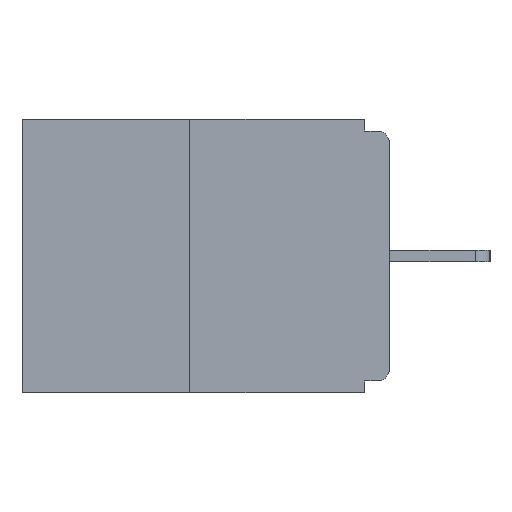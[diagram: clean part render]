
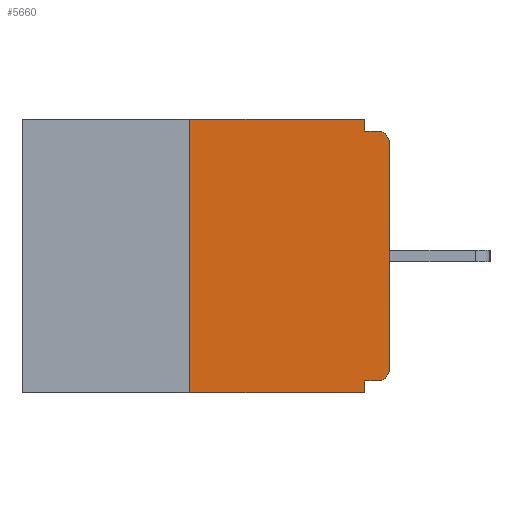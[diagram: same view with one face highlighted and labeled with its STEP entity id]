
A CAD part, left-side view. The second image highlights one B-rep face of the part: STEP entity #5660.
In plain terms, the highlighted planar face has unit normal (-1, 0, 0).
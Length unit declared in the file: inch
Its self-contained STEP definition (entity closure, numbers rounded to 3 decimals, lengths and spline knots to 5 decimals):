
#45 = ORIENTED_EDGE ( 'NONE', *, *, #11676, .F. ) ;
#504 = VECTOR ( 'NONE', #8665, 39.37008 ) ;
#790 = DIRECTION ( 'NONE',  ( 0., -1., 0. ) ) ;
#832 = CARTESIAN_POINT ( 'NONE',  ( 0., 0.46, 0. ) ) ;
#844 = CARTESIAN_POINT ( 'NONE',  ( 0., 0.031, -0.343 ) ) ;
#902 = PLANE ( 'NONE',  #1967 ) ;
#1046 = VERTEX_POINT ( 'NONE', #8245 ) ;
#1131 = LINE ( 'NONE', #14130, #15186 ) ;
#1216 = ORIENTED_EDGE ( 'NONE', *, *, #13481, .F. ) ;
#1357 = CARTESIAN_POINT ( 'NONE',  ( 0., 0.031, -0.015 ) ) ;
#1545 = ORIENTED_EDGE ( 'NONE', *, *, #9710, .T. ) ;
#1563 = LINE ( 'NONE', #6252, #3145 ) ;
#1680 = EDGE_CURVE ( 'NONE', #12583, #5940, #13555, .T. ) ;
#1902 = CARTESIAN_POINT ( 'NONE',  ( 0., 0.25, -0.343 ) ) ;
#1910 = CARTESIAN_POINT ( 'NONE',  ( 0., 0.015, -0.015 ) ) ;
#1967 = AXIS2_PLACEMENT_3D ( 'NONE', #832, #1994, #3025 ) ;
#1988 = CARTESIAN_POINT ( 'NONE',  ( 0., 0., 0. ) ) ;
#1994 = DIRECTION ( 'NONE',  ( 1., 0., 0. ) ) ;
#2125 = DIRECTION ( 'NONE',  ( 0., 0., -1. ) ) ;
#2449 = VECTOR ( 'NONE', #7074, 39.37008 ) ;
#2822 = CARTESIAN_POINT ( 'NONE',  ( 0., 0.031, 0. ) ) ;
#3025 = DIRECTION ( 'NONE',  ( 0., 0., -1. ) ) ;
#3145 = VECTOR ( 'NONE', #12181, 39.37008 ) ;
#3301 = DIRECTION ( 'NONE',  ( -1., 0., 0. ) ) ;
#3336 = DIRECTION ( 'NONE',  ( 0., 0., -1. ) ) ;
#3425 = CARTESIAN_POINT ( 'NONE',  ( 0., 0., -0.03 ) ) ;
#3451 = DIRECTION ( 'NONE',  ( -1., 0., 0. ) ) ;
#3454 = EDGE_CURVE ( 'NONE', #7929, #8528, #11336, .T. ) ;
#3764 = VECTOR ( 'NONE', #10218, 39.37008 ) ;
#3963 = VERTEX_POINT ( 'NONE', #1902 ) ;
#4091 = CARTESIAN_POINT ( 'NONE',  ( 0., 0.031, 0. ) ) ;
#4121 = CARTESIAN_POINT ( 'NONE',  ( 0., 0.46, 0. ) ) ;
#4866 = CARTESIAN_POINT ( 'NONE',  ( 0., 0.015, -0.328 ) ) ;
#4900 = CIRCLE ( 'NONE', #6665, 0.015 ) ;
#5142 = VERTEX_POINT ( 'NONE', #1910 ) ;
#5660 = ADVANCED_FACE ( 'NONE', ( #11461 ), #902, .F. ) ;
#5722 = CARTESIAN_POINT ( 'NONE',  ( 0., 0.015, -0.313 ) ) ;
#5940 = VERTEX_POINT ( 'NONE', #1357 ) ;
#6252 = CARTESIAN_POINT ( 'NONE',  ( 0., 0.25, 0. ) ) ;
#6557 = CARTESIAN_POINT ( 'NONE',  ( 0., 0.031, -0.328 ) ) ;
#6665 = AXIS2_PLACEMENT_3D ( 'NONE', #9496, #3451, #2125 ) ;
#7074 = DIRECTION ( 'NONE',  ( 0., 0., 1. ) ) ;
#7313 = VECTOR ( 'NONE', #3336, 39.37008 ) ;
#7446 = VECTOR ( 'NONE', #790, 39.37008 ) ;
#7634 = ORIENTED_EDGE ( 'NONE', *, *, #10480, .T. ) ;
#7929 = VERTEX_POINT ( 'NONE', #6557 ) ;
#8245 = CARTESIAN_POINT ( 'NONE',  ( 0., 0.25, 0. ) ) ;
#8295 = ORIENTED_EDGE ( 'NONE', *, *, #1680, .F. ) ;
#8528 = VERTEX_POINT ( 'NONE', #12852 ) ;
#8605 = EDGE_CURVE ( 'NONE', #11984, #7929, #9116, .T. ) ;
#8665 = DIRECTION ( 'NONE',  ( 0., -1., 0. ) ) ;
#8825 = LINE ( 'NONE', #4121, #504 ) ;
#9088 = DIRECTION ( 'NONE',  ( 0., 0., -1. ) ) ;
#9116 = LINE ( 'NONE', #11451, #3764 ) ;
#9176 = DIRECTION ( 'NONE',  ( 0., 0., -1. ) ) ;
#9295 = AXIS2_PLACEMENT_3D ( 'NONE', #5722, #3301, #9176 ) ;
#9426 = LINE ( 'NONE', #1988, #2449 ) ;
#9496 = CARTESIAN_POINT ( 'NONE',  ( 0., 0.015, -0.03 ) ) ;
#9510 = VECTOR ( 'NONE', #9088, 39.37008 ) ;
#9710 = EDGE_CURVE ( 'NONE', #11984, #9798, #10054, .T. ) ;
#9798 = VERTEX_POINT ( 'NONE', #10297 ) ;
#10054 = CIRCLE ( 'NONE', #9295, 0.015 ) ;
#10218 = DIRECTION ( 'NONE',  ( 0., 1., 0. ) ) ;
#10297 = CARTESIAN_POINT ( 'NONE',  ( 0., 0., -0.313 ) ) ;
#10307 = ORIENTED_EDGE ( 'NONE', *, *, #12249, .T. ) ;
#10351 = CARTESIAN_POINT ( 'NONE',  ( 0., 0., -0.015 ) ) ;
#10467 = DIRECTION ( 'NONE',  ( 0., -1., 0. ) ) ;
#10480 = EDGE_CURVE ( 'NONE', #3963, #8528, #1131, .T. ) ;
#11258 = ORIENTED_EDGE ( 'NONE', *, *, #8605, .F. ) ;
#11336 = LINE ( 'NONE', #844, #7313 ) ;
#11451 = CARTESIAN_POINT ( 'NONE',  ( 0., 0., -0.328 ) ) ;
#11461 = FACE_OUTER_BOUND ( 'NONE', #15269, .T. ) ;
#11676 = EDGE_CURVE ( 'NONE', #3963, #1046, #1563, .T. ) ;
#11862 = ORIENTED_EDGE ( 'NONE', *, *, #3454, .F. ) ;
#11984 = VERTEX_POINT ( 'NONE', #4866 ) ;
#12181 = DIRECTION ( 'NONE',  ( 0., 0., 1. ) ) ;
#12249 = EDGE_CURVE ( 'NONE', #13649, #5142, #4900, .T. ) ;
#12583 = VERTEX_POINT ( 'NONE', #4091 ) ;
#12814 = ORIENTED_EDGE ( 'NONE', *, *, #15446, .F. ) ;
#12852 = CARTESIAN_POINT ( 'NONE',  ( 0., 0.031, -0.343 ) ) ;
#13067 = ORIENTED_EDGE ( 'NONE', *, *, #13421, .T. ) ;
#13421 = EDGE_CURVE ( 'NONE', #9798, #13649, #9426, .T. ) ;
#13481 = EDGE_CURVE ( 'NONE', #5940, #5142, #15258, .T. ) ;
#13555 = LINE ( 'NONE', #2822, #9510 ) ;
#13649 = VERTEX_POINT ( 'NONE', #3425 ) ;
#14130 = CARTESIAN_POINT ( 'NONE',  ( 0., 0.46, -0.343 ) ) ;
#15186 = VECTOR ( 'NONE', #10467, 39.37008 ) ;
#15258 = LINE ( 'NONE', #10351, #7446 ) ;
#15269 = EDGE_LOOP ( 'NONE', ( #12814, #45, #7634, #11862, #11258, #1545, #13067, #10307, #1216, #8295 ) ) ;
#15446 = EDGE_CURVE ( 'NONE', #1046, #12583, #8825, .T. ) ;
